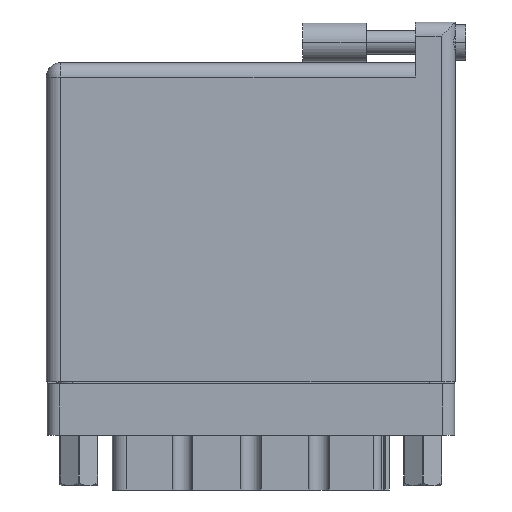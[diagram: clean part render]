
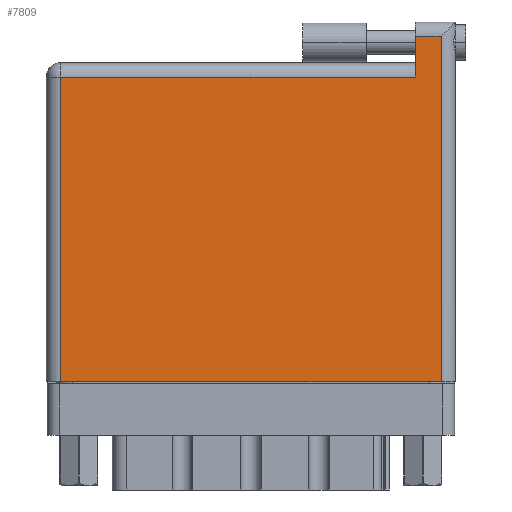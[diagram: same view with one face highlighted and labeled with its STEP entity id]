
A CAD part, front view. The second image highlights one B-rep face of the part: STEP entity #7809.
In plain terms, the highlighted face is planar.
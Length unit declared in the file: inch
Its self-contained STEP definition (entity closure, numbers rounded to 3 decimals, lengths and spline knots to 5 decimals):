
#220 = EDGE_CURVE ( 'NONE', #17572, #44136, #10240, .T. ) ;
#817 = CARTESIAN_POINT ( 'NONE',  ( 1.938, 1.766, 0. ) ) ;
#862 = DIRECTION ( 'NONE',  ( -1., 0., 0. ) ) ;
#1770 = EDGE_CURVE ( 'NONE', #40603, #28367, #29771, .T. ) ;
#4167 = VECTOR ( 'NONE', #44508, 39.37008 ) ;
#4423 = DIRECTION ( 'NONE',  ( -1., 0., 0. ) ) ;
#5848 = VERTEX_POINT ( 'NONE', #28940 ) ;
#6051 = ORIENTED_EDGE ( 'NONE', *, *, #220, .T. ) ;
#7654 = EDGE_CURVE ( 'NONE', #44136, #5848, #49161, .T. ) ;
#7809 = ADVANCED_FACE ( 'NONE', ( #8817 ), #22162, .F. ) ;
#8817 = FACE_OUTER_BOUND ( 'NONE', #28305, .T. ) ;
#10240 = LINE ( 'NONE', #17654, #32505 ) ;
#11935 = LINE ( 'NONE', #35213, #45057 ) ;
#12107 = ORIENTED_EDGE ( 'NONE', *, *, #27450, .T. ) ;
#15102 = CARTESIAN_POINT ( 'NONE',  ( 0.07, 0., 0. ) ) ;
#15688 = CARTESIAN_POINT ( 'NONE',  ( 0., 1.496, 0. ) ) ;
#16050 = AXIS2_PLACEMENT_3D ( 'NONE', #29912, #48904, #25874 ) ;
#17572 = VERTEX_POINT ( 'NONE', #15102 ) ;
#17654 = CARTESIAN_POINT ( 'NONE',  ( 0., 0., 0. ) ) ;
#17838 = VECTOR ( 'NONE', #27757, 39.37008 ) ;
#19506 = VECTOR ( 'NONE', #862, 39.37008 ) ;
#19835 = ORIENTED_EDGE ( 'NONE', *, *, #22815, .T. ) ;
#21036 = LINE ( 'NONE', #25498, #4167 ) ;
#22162 = PLANE ( 'NONE',  #16050 ) ;
#22728 = CARTESIAN_POINT ( 'NONE',  ( 1.811, 1.496, 0. ) ) ;
#22815 = EDGE_CURVE ( 'NONE', #28367, #17572, #21036, .T. ) ;
#24812 = EDGE_CURVE ( 'NONE', #5848, #38676, #34446, .T. ) ;
#25498 = CARTESIAN_POINT ( 'NONE',  ( 0.07, 0., 0. ) ) ;
#25874 = DIRECTION ( 'NONE',  ( -1., 0., 0. ) ) ;
#26246 = ORIENTED_EDGE ( 'NONE', *, *, #1770, .T. ) ;
#27450 = EDGE_CURVE ( 'NONE', #38676, #40603, #11935, .T. ) ;
#27615 = DIRECTION ( 'NONE',  ( 0., -1., 0. ) ) ;
#27757 = DIRECTION ( 'NONE',  ( 0., 1., 0. ) ) ;
#28305 = EDGE_LOOP ( 'NONE', ( #6051, #40439, #29812, #12107, #26246, #19835 ) ) ;
#28367 = VERTEX_POINT ( 'NONE', #29080 ) ;
#28806 = DIRECTION ( 'NONE',  ( 1., 0., 0. ) ) ;
#28940 = CARTESIAN_POINT ( 'NONE',  ( 1.938, 1.696, 0. ) ) ;
#29080 = CARTESIAN_POINT ( 'NONE',  ( 0.07, 1.496, 0. ) ) ;
#29771 = LINE ( 'NONE', #15688, #19506 ) ;
#29812 = ORIENTED_EDGE ( 'NONE', *, *, #24812, .T. ) ;
#29912 = CARTESIAN_POINT ( 'NONE',  ( 0., 1.566, 0. ) ) ;
#32505 = VECTOR ( 'NONE', #28806, 39.37008 ) ;
#34446 = LINE ( 'NONE', #46685, #44063 ) ;
#35213 = CARTESIAN_POINT ( 'NONE',  ( 1.811, 1.766, 0. ) ) ;
#38676 = VERTEX_POINT ( 'NONE', #46674 ) ;
#40439 = ORIENTED_EDGE ( 'NONE', *, *, #7654, .T. ) ;
#40603 = VERTEX_POINT ( 'NONE', #22728 ) ;
#44063 = VECTOR ( 'NONE', #4423, 39.37008 ) ;
#44136 = VERTEX_POINT ( 'NONE', #45464 ) ;
#44508 = DIRECTION ( 'NONE',  ( 0., -1., 0. ) ) ;
#45057 = VECTOR ( 'NONE', #27615, 39.37008 ) ;
#45464 = CARTESIAN_POINT ( 'NONE',  ( 1.938, 0., 0. ) ) ;
#46674 = CARTESIAN_POINT ( 'NONE',  ( 1.811, 1.696, 0. ) ) ;
#46685 = CARTESIAN_POINT ( 'NONE',  ( 0., 1.696, 0. ) ) ;
#48904 = DIRECTION ( 'NONE',  ( 0., 0., -1. ) ) ;
#49161 = LINE ( 'NONE', #817, #17838 ) ;
